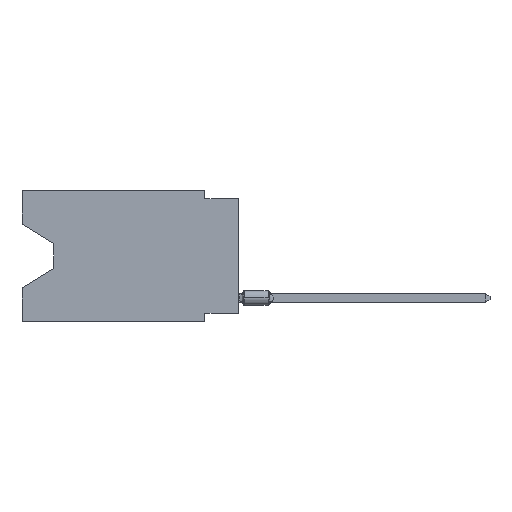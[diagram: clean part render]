
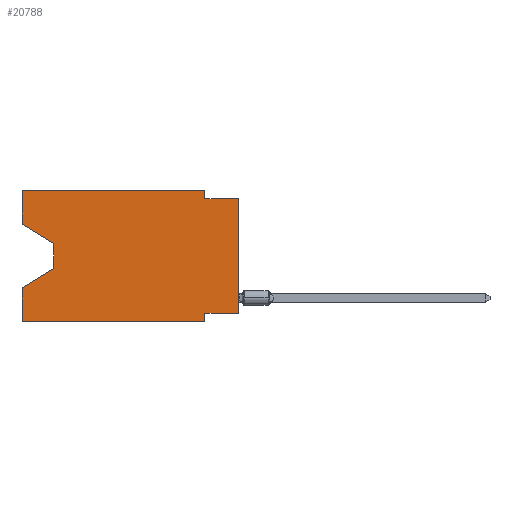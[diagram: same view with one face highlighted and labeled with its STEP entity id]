
A CAD part, left-side view. The second image highlights one B-rep face of the part: STEP entity #20788.
In plain terms, the highlighted planar face has unit normal (-1, 0, 0).
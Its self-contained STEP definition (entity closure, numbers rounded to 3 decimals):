
#717 = DIRECTION ( 'NONE',  ( 0., -1., 0. ) ) ;
#840 = LINE ( 'NONE', #25500, #21225 ) ;
#1013 = ORIENTED_EDGE ( 'NONE', *, *, #6048, .F. ) ;
#1382 = VECTOR ( 'NONE', #16081, 1000. ) ;
#1529 = CARTESIAN_POINT ( 'NONE',  ( 0., 16.383, -2.546 ) ) ;
#1641 = VERTEX_POINT ( 'NONE', #24058 ) ;
#2743 = VERTEX_POINT ( 'NONE', #1529 ) ;
#4589 = DIRECTION ( 'NONE',  ( 0., 0., 1. ) ) ;
#4687 = CARTESIAN_POINT ( 'NONE',  ( 0., 2.54, 0. ) ) ;
#5089 = CARTESIAN_POINT ( 'NONE',  ( 0., 16.383, -9.906 ) ) ;
#5188 = VECTOR ( 'NONE', #4589, 1000. ) ;
#5279 = VECTOR ( 'NONE', #8510, 1000. ) ;
#5405 = CARTESIAN_POINT ( 'NONE',  ( 0., 13.97, -5.893 ) ) ;
#5504 = CARTESIAN_POINT ( 'NONE',  ( 0., 16.383, 0. ) ) ;
#5579 = LINE ( 'NONE', #21794, #23234 ) ;
#5732 = VECTOR ( 'NONE', #24386, 1000. ) ;
#6025 = PLANE ( 'NONE',  #9849 ) ;
#6048 = EDGE_CURVE ( 'NONE', #1641, #15582, #6955, .T. ) ;
#6129 = ORIENTED_EDGE ( 'NONE', *, *, #24967, .F. ) ;
#6132 = DIRECTION ( 'NONE',  ( 0., -1., 0. ) ) ;
#6249 = ORIENTED_EDGE ( 'NONE', *, *, #9828, .T. ) ;
#6274 = EDGE_CURVE ( 'NONE', #2743, #16144, #24357, .T. ) ;
#6397 = CARTESIAN_POINT ( 'NONE',  ( 0., 16.383, 0. ) ) ;
#6445 = ORIENTED_EDGE ( 'NONE', *, *, #13472, .F. ) ;
#6660 = LINE ( 'NONE', #14695, #20718 ) ;
#6955 = LINE ( 'NONE', #13132, #21237 ) ;
#7050 = ORIENTED_EDGE ( 'NONE', *, *, #19311, .T. ) ;
#7145 = EDGE_CURVE ( 'NONE', #10743, #25419, #7915, .T. ) ;
#7291 = DIRECTION ( 'NONE',  ( 0., 0.855, -0.519 ) ) ;
#7471 = CARTESIAN_POINT ( 'NONE',  ( 0., 2.54, -0.635 ) ) ;
#7563 = CARTESIAN_POINT ( 'NONE',  ( 0., 13.97, -5.893 ) ) ;
#7915 = LINE ( 'NONE', #18083, #1382 ) ;
#8510 = DIRECTION ( 'NONE',  ( 0., 0., 1. ) ) ;
#8719 = DIRECTION ( 'NONE',  ( 0., 0., -1. ) ) ;
#8776 = VERTEX_POINT ( 'NONE', #5405 ) ;
#8872 = VECTOR ( 'NONE', #20361, 1000. ) ;
#9093 = EDGE_CURVE ( 'NONE', #16144, #8776, #21191, .T. ) ;
#9423 = CARTESIAN_POINT ( 'NONE',  ( 0., 2.54, -9.906 ) ) ;
#9828 = EDGE_CURVE ( 'NONE', #24442, #18180, #6660, .T. ) ;
#9849 = AXIS2_PLACEMENT_3D ( 'NONE', #9896, #22654, #24521 ) ;
#9896 = CARTESIAN_POINT ( 'NONE',  ( 0., 16.383, 0. ) ) ;
#10231 = DIRECTION ( 'NONE',  ( 0., 0., -1. ) ) ;
#10743 = VERTEX_POINT ( 'NONE', #6397 ) ;
#11015 = ORIENTED_EDGE ( 'NONE', *, *, #17821, .F. ) ;
#11233 = ORIENTED_EDGE ( 'NONE', *, *, #21720, .F. ) ;
#12180 = CARTESIAN_POINT ( 'NONE',  ( 0., 16.383, -7.36 ) ) ;
#13132 = CARTESIAN_POINT ( 'NONE',  ( 0., 0., -9.271 ) ) ;
#13472 = EDGE_CURVE ( 'NONE', #2743, #10743, #17687, .T. ) ;
#14323 = CARTESIAN_POINT ( 'NONE',  ( 0., 16.383, -2.546 ) ) ;
#14518 = CARTESIAN_POINT ( 'NONE',  ( 0., 2.54, -9.906 ) ) ;
#14594 = FACE_OUTER_BOUND ( 'NONE', #18737, .T. ) ;
#14614 = CARTESIAN_POINT ( 'NONE',  ( 0., 13.97, -4.013 ) ) ;
#14695 = CARTESIAN_POINT ( 'NONE',  ( 0., 16.383, -9.906 ) ) ;
#14776 = CARTESIAN_POINT ( 'NONE',  ( 0., 16.383, 0. ) ) ;
#15061 = CARTESIAN_POINT ( 'NONE',  ( 0., 0., 0. ) ) ;
#15171 = VERTEX_POINT ( 'NONE', #7471 ) ;
#15382 = ORIENTED_EDGE ( 'NONE', *, *, #7145, .F. ) ;
#15582 = VERTEX_POINT ( 'NONE', #16957 ) ;
#15781 = CARTESIAN_POINT ( 'NONE',  ( 0., 0., -0.635 ) ) ;
#16081 = DIRECTION ( 'NONE',  ( 0., -1., 0. ) ) ;
#16144 = VERTEX_POINT ( 'NONE', #22575 ) ;
#16768 = VECTOR ( 'NONE', #10231, 1000. ) ;
#16773 = LINE ( 'NONE', #14518, #16768 ) ;
#16957 = CARTESIAN_POINT ( 'NONE',  ( 0., 2.54, -9.271 ) ) ;
#17590 = LINE ( 'NONE', #7563, #23260 ) ;
#17646 = VECTOR ( 'NONE', #8719, 1000. ) ;
#17687 = LINE ( 'NONE', #5504, #5732 ) ;
#17720 = ORIENTED_EDGE ( 'NONE', *, *, #19440, .T. ) ;
#17821 = EDGE_CURVE ( 'NONE', #15171, #23464, #840, .T. ) ;
#18083 = CARTESIAN_POINT ( 'NONE',  ( 0., 16.383, 0. ) ) ;
#18180 = VERTEX_POINT ( 'NONE', #9423 ) ;
#18737 = EDGE_LOOP ( 'NONE', ( #21065, #26293, #17720, #11233, #6249, #6129, #1013, #7050, #11015, #20289, #15382, #6445 ) ) ;
#19022 = EDGE_CURVE ( 'NONE', #25419, #15171, #5579, .T. ) ;
#19222 = LINE ( 'NONE', #15061, #5279 ) ;
#19311 = EDGE_CURVE ( 'NONE', #1641, #23464, #19222, .T. ) ;
#19440 = EDGE_CURVE ( 'NONE', #8776, #21198, #17590, .T. ) ;
#20289 = ORIENTED_EDGE ( 'NONE', *, *, #19022, .F. ) ;
#20361 = DIRECTION ( 'NONE',  ( 0., -0.855, -0.519 ) ) ;
#20718 = VECTOR ( 'NONE', #6132, 1000. ) ;
#20788 = ADVANCED_FACE ( 'NONE', ( #14594 ), #6025, .F. ) ;
#21065 = ORIENTED_EDGE ( 'NONE', *, *, #6274, .T. ) ;
#21191 = LINE ( 'NONE', #14614, #17646 ) ;
#21198 = VERTEX_POINT ( 'NONE', #12180 ) ;
#21225 = VECTOR ( 'NONE', #717, 1000. ) ;
#21237 = VECTOR ( 'NONE', #21301, 1000. ) ;
#21301 = DIRECTION ( 'NONE',  ( 0., 1., 0. ) ) ;
#21720 = EDGE_CURVE ( 'NONE', #24442, #21198, #24050, .T. ) ;
#21794 = CARTESIAN_POINT ( 'NONE',  ( 0., 2.54, 0. ) ) ;
#21921 = DIRECTION ( 'NONE',  ( 0., 0., -1. ) ) ;
#22575 = CARTESIAN_POINT ( 'NONE',  ( 0., 13.97, -4.013 ) ) ;
#22654 = DIRECTION ( 'NONE',  ( 1., 0., 0. ) ) ;
#23234 = VECTOR ( 'NONE', #21921, 1000. ) ;
#23260 = VECTOR ( 'NONE', #7291, 1000. ) ;
#23464 = VERTEX_POINT ( 'NONE', #15781 ) ;
#24050 = LINE ( 'NONE', #14776, #5188 ) ;
#24058 = CARTESIAN_POINT ( 'NONE',  ( 0., 0., -9.271 ) ) ;
#24357 = LINE ( 'NONE', #14323, #8872 ) ;
#24386 = DIRECTION ( 'NONE',  ( 0., 0., 1. ) ) ;
#24442 = VERTEX_POINT ( 'NONE', #5089 ) ;
#24521 = DIRECTION ( 'NONE',  ( 0., 0., -1. ) ) ;
#24967 = EDGE_CURVE ( 'NONE', #15582, #18180, #16773, .T. ) ;
#25419 = VERTEX_POINT ( 'NONE', #4687 ) ;
#25500 = CARTESIAN_POINT ( 'NONE',  ( 0., 0., -0.635 ) ) ;
#26293 = ORIENTED_EDGE ( 'NONE', *, *, #9093, .T. ) ;
